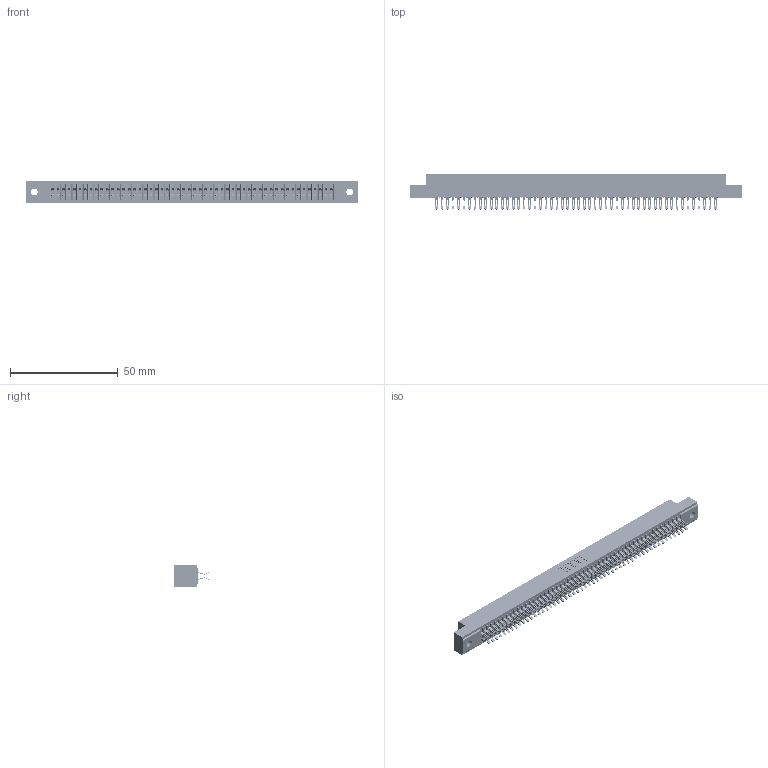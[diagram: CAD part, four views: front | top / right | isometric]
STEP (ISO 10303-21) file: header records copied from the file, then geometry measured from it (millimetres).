
FILE_DESCRIPTION (( 'STEP AP203' ), '1' );
FILE_NAME ('391-104-555-202.STEP', '2018-08-09T20:26:11', ( '' ), ( '' ), 'SwSTEP 2.0', 'SolidWorks 2016', '' );
FILE_SCHEMA (( 'CONFIG_CONTROL_DESIGN' ));
Length unit declared in the file: inch
Products named in the file (3): 341 Part_.128 (3.25) Dia Mounting Holes; 341-292-001_341-292-155; 391-104-555-202
Assembly tree (105 placements, depth 2):
  391-104-555-202
    341 Part_.128 (3.25) Dia Mounting Holes
    341-292-001_341-292-155  x104
Bounding box: 154.31 x 16.31 x 10.16 mm (x, y, z)
Volume: 11495.5 mm3; surface area: 21319.6 mm2
Topology: 105 solids, 105 shells, 8228 faces, 24600 edges, 16014 vertices
Faces by surface type: plane 4436, cylinder 3584, sphere 106, torus 102
Entity records: 62071 total; most frequent: CARTESIAN_POINT 10334, ORIENTED_EDGE 10260, DIRECTION 10012, EDGE_CURVE 5130, LINE 4140, VECTOR 4140, VERTEX_POINT 3242, AXIS2_PLACEMENT_3D 2936
